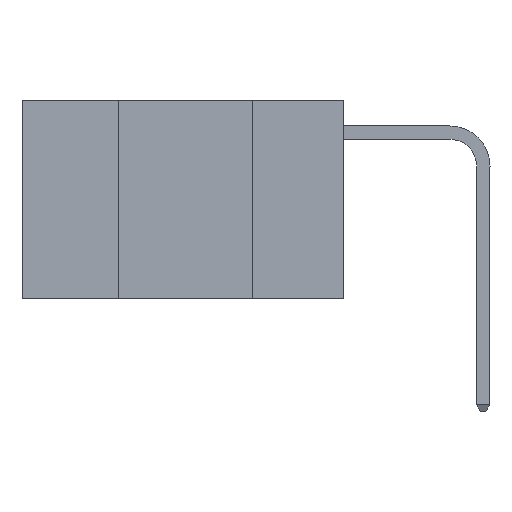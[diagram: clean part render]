
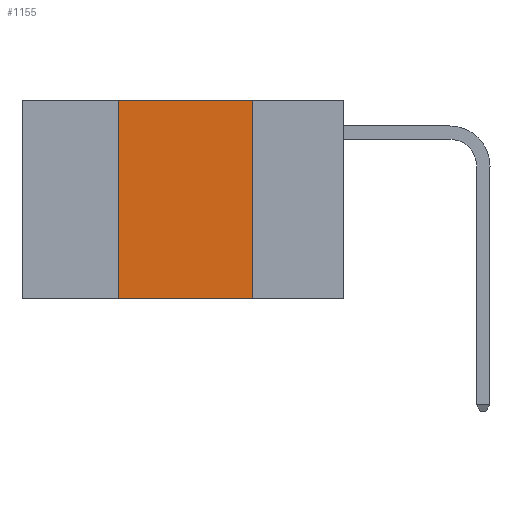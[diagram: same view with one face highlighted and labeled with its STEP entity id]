
A CAD part, left-side view. The second image highlights one B-rep face of the part: STEP entity #1155.
In plain terms, the highlighted planar face has unit normal (-1, 0, 0).
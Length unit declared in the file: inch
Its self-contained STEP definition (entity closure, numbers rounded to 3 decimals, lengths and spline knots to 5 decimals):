
#194 = DIRECTION ( 'NONE',  ( 1., 0., 0. ) ) ;
#320 = AXIS2_PLACEMENT_3D ( 'NONE', #5785, #194, #1274 ) ;
#1155 = ADVANCED_FACE ( 'NONE', ( #5220 ), #7867, .F. ) ;
#1274 = DIRECTION ( 'NONE',  ( 0., 0., -1. ) ) ;
#1574 = CARTESIAN_POINT ( 'NONE',  ( 0., 0.6, -0.37 ) ) ;
#2069 = VERTEX_POINT ( 'NONE', #2698 ) ;
#2327 = EDGE_LOOP ( 'NONE', ( #3375, #9491, #3295, #4203 ) ) ;
#2698 = CARTESIAN_POINT ( 'NONE',  ( 0., 0.42, 0. ) ) ;
#2721 = CARTESIAN_POINT ( 'NONE',  ( 0., 0.6, 0. ) ) ;
#2750 = CARTESIAN_POINT ( 'NONE',  ( 0., 0.42, -0.37 ) ) ;
#3140 = DIRECTION ( 'NONE',  ( 0., -1., 0. ) ) ;
#3295 = ORIENTED_EDGE ( 'NONE', *, *, #4777, .F. ) ;
#3375 = ORIENTED_EDGE ( 'NONE', *, *, #5194, .F. ) ;
#3761 = VECTOR ( 'NONE', #6320, 39.37008 ) ;
#3830 = LINE ( 'NONE', #6419, #3761 ) ;
#3873 = EDGE_CURVE ( 'NONE', #2069, #10108, #9262, .T. ) ;
#4171 = VERTEX_POINT ( 'NONE', #7462 ) ;
#4203 = ORIENTED_EDGE ( 'NONE', *, *, #10504, .T. ) ;
#4777 = EDGE_CURVE ( 'NONE', #8125, #2069, #5884, .T. ) ;
#5149 = DIRECTION ( 'NONE',  ( 0., -1., 0. ) ) ;
#5194 = EDGE_CURVE ( 'NONE', #10108, #4171, #3830, .T. ) ;
#5220 = FACE_OUTER_BOUND ( 'NONE', #2327, .T. ) ;
#5338 = CARTESIAN_POINT ( 'NONE',  ( 0., 0.17, 0. ) ) ;
#5776 = VECTOR ( 'NONE', #9690, 39.37008 ) ;
#5785 = CARTESIAN_POINT ( 'NONE',  ( 0., 0.6, 0. ) ) ;
#5884 = LINE ( 'NONE', #9725, #5776 ) ;
#6320 = DIRECTION ( 'NONE',  ( 0., 0., -1. ) ) ;
#6419 = CARTESIAN_POINT ( 'NONE',  ( 0., 0.17, 0. ) ) ;
#7462 = CARTESIAN_POINT ( 'NONE',  ( 0., 0.17, -0.37 ) ) ;
#7867 = PLANE ( 'NONE',  #320 ) ;
#8125 = VERTEX_POINT ( 'NONE', #2750 ) ;
#8515 = VECTOR ( 'NONE', #5149, 39.37008 ) ;
#8779 = LINE ( 'NONE', #1574, #8515 ) ;
#9224 = VECTOR ( 'NONE', #3140, 39.37008 ) ;
#9262 = LINE ( 'NONE', #2721, #9224 ) ;
#9491 = ORIENTED_EDGE ( 'NONE', *, *, #3873, .F. ) ;
#9690 = DIRECTION ( 'NONE',  ( 0., 0., 1. ) ) ;
#9725 = CARTESIAN_POINT ( 'NONE',  ( 0., 0.42, 0. ) ) ;
#10108 = VERTEX_POINT ( 'NONE', #5338 ) ;
#10504 = EDGE_CURVE ( 'NONE', #8125, #4171, #8779, .T. ) ;
